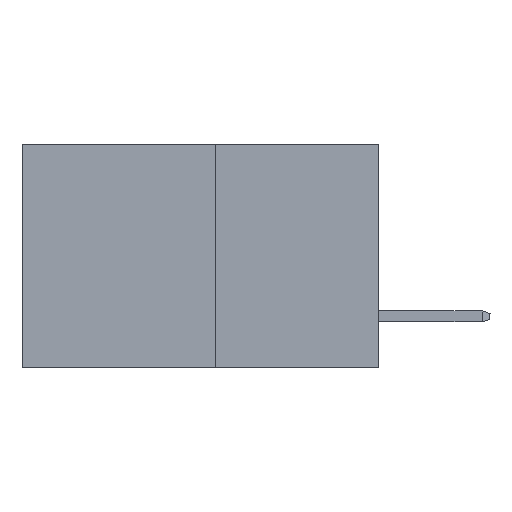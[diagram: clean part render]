
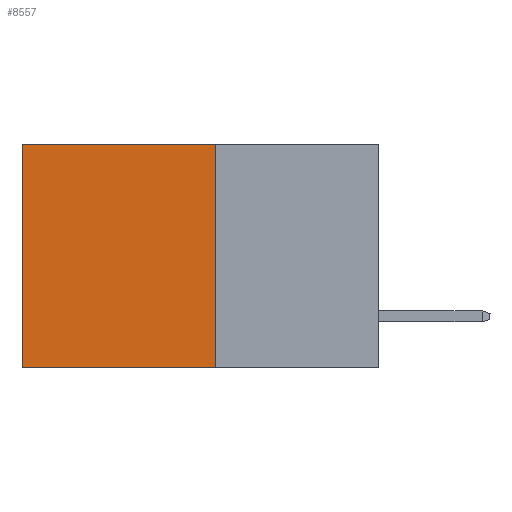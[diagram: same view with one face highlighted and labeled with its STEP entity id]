
A CAD part, left-side view. The second image highlights one B-rep face of the part: STEP entity #8557.
In plain terms, the highlighted planar face has unit normal (-1, 0, 0).
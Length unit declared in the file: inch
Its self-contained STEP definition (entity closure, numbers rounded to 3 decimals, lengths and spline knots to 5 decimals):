
#457 = EDGE_CURVE ( 'NONE', #2562, #12261, #13325, .T. ) ;
#487 = CARTESIAN_POINT ( 'NONE',  ( 0.277, 0.27, 0. ) ) ;
#1511 = CARTESIAN_POINT ( 'NONE',  ( 0.277, 0.59, 0. ) ) ;
#1794 = ORIENTED_EDGE ( 'NONE', *, *, #457, .T. ) ;
#2366 = ORIENTED_EDGE ( 'NONE', *, *, #16747, .T. ) ;
#2562 = VERTEX_POINT ( 'NONE', #487 ) ;
#3607 = CARTESIAN_POINT ( 'NONE',  ( 0.277, 0.59, -0.37 ) ) ;
#4075 = EDGE_LOOP ( 'NONE', ( #2366, #25607, #18581, #1794 ) ) ;
#6954 = LINE ( 'NONE', #24885, #11835 ) ;
#7326 = EDGE_CURVE ( 'NONE', #2562, #25667, #6954, .T. ) ;
#7551 = FACE_OUTER_BOUND ( 'NONE', #4075, .T. ) ;
#7624 = CARTESIAN_POINT ( 'NONE',  ( 0.277, 0.27, -0.37 ) ) ;
#8557 = ADVANCED_FACE ( 'NONE', ( #7551 ), #16206, .F. ) ;
#9602 = CARTESIAN_POINT ( 'NONE',  ( 0.277, 0.27, -0.37 ) ) ;
#9702 = DIRECTION ( 'NONE',  ( 0., 1., 0. ) ) ;
#10098 = DIRECTION ( 'NONE',  ( 1., 0., 0. ) ) ;
#11260 = LINE ( 'NONE', #3607, #22197 ) ;
#11835 = VECTOR ( 'NONE', #16701, 39.37008 ) ;
#12261 = VERTEX_POINT ( 'NONE', #1511 ) ;
#13325 = LINE ( 'NONE', #18828, #24275 ) ;
#16206 = PLANE ( 'NONE',  #21063 ) ;
#16701 = DIRECTION ( 'NONE',  ( 0., 0., -1. ) ) ;
#16747 = EDGE_CURVE ( 'NONE', #12261, #19476, #11260, .T. ) ;
#18581 = ORIENTED_EDGE ( 'NONE', *, *, #7326, .F. ) ;
#18828 = CARTESIAN_POINT ( 'NONE',  ( 0.277, 0.27, 0. ) ) ;
#19476 = VERTEX_POINT ( 'NONE', #21683 ) ;
#19564 = EDGE_CURVE ( 'NONE', #25667, #19476, #20118, .T. ) ;
#20118 = LINE ( 'NONE', #7624, #25560 ) ;
#20687 = DIRECTION ( 'NONE',  ( 0., 0., -1. ) ) ;
#20764 = DIRECTION ( 'NONE',  ( 0., 1., 0. ) ) ;
#21063 = AXIS2_PLACEMENT_3D ( 'NONE', #26434, #10098, #24477 ) ;
#21683 = CARTESIAN_POINT ( 'NONE',  ( 0.277, 0.59, -0.37 ) ) ;
#22197 = VECTOR ( 'NONE', #20687, 39.37008 ) ;
#24275 = VECTOR ( 'NONE', #20764, 39.37008 ) ;
#24477 = DIRECTION ( 'NONE',  ( 0., 0., -1. ) ) ;
#24885 = CARTESIAN_POINT ( 'NONE',  ( 0.277, 0.27, -0.37 ) ) ;
#25560 = VECTOR ( 'NONE', #9702, 39.37008 ) ;
#25607 = ORIENTED_EDGE ( 'NONE', *, *, #19564, .F. ) ;
#25667 = VERTEX_POINT ( 'NONE', #9602 ) ;
#26434 = CARTESIAN_POINT ( 'NONE',  ( 0.277, 0.27, -0.37 ) ) ;
